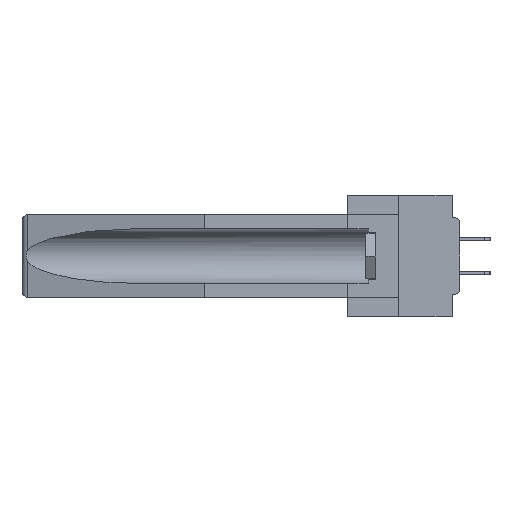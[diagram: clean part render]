
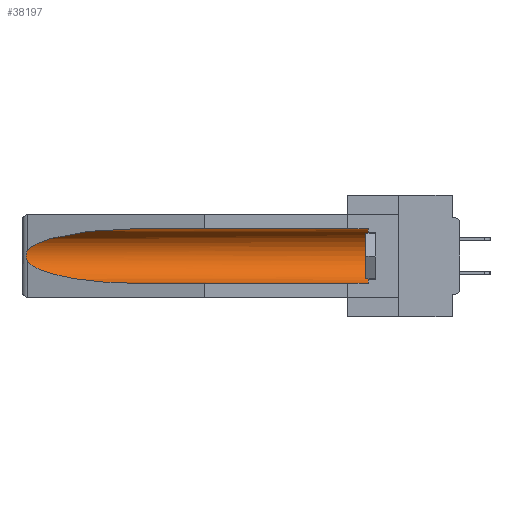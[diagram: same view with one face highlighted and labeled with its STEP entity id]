
A CAD part, left-side view. The second image highlights one B-rep face of the part: STEP entity #38197.
In plain terms, the highlighted cylindrical face has radius 2.857 mm (diameter 5.715 mm), a partial arc.
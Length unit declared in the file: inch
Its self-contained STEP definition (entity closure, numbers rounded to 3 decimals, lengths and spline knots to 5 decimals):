
#749 = CARTESIAN_POINT ( 'NONE',  ( 0.155, 0.126, -0.059 ) ) ;
#2860 = CARTESIAN_POINT ( 'NONE',  ( 0.25451, 1.48313, -0.09465 ) ) ;
#5526 = CARTESIAN_POINT ( 'NONE',  ( 0.2675, 1.53308, -0.16763 ) ) ;
#6172 = CARTESIAN_POINT ( 'NONE',  ( 0.26537, 1.52718, -0.14972 ) ) ;
#7469 = CARTESIAN_POINT ( 'NONE',  ( 0.155, 0.126, -0.1715 ) ) ;
#7649 = ORIENTED_EDGE ( 'NONE', *, *, #25995, .T. ) ;
#9247 = FACE_OUTER_BOUND ( 'NONE', #11034, .T. ) ;
#9677 = EDGE_CURVE ( 'NONE', #30293, #32261, #29166, .T. ) ;
#11034 = EDGE_LOOP ( 'NONE', ( #7649, #43003, #21508, #26777, #19174, #17220 ) ) ;
#11439 = VERTEX_POINT ( 'NONE', #749 ) ;
#12349 = VERTEX_POINT ( 'NONE', #33799 ) ;
#13702 = CARTESIAN_POINT ( 'NONE',  ( 0.155, 1.07973, -0.284 ) ) ;
#16605 = VERTEX_POINT ( 'NONE', #41737 ) ;
#17220 = ORIENTED_EDGE ( 'NONE', *, *, #38692, .T. ) ;
#17926 = DIRECTION ( 'NONE',  ( 0., -1., 0. ) ) ;
#17949 = AXIS2_PLACEMENT_3D ( 'NONE', #36084, #39409, #43514 ) ;
#19174 = ORIENTED_EDGE ( 'NONE', *, *, #40276, .T. ) ;
#19902 = CARTESIAN_POINT ( 'NONE',  ( 0.26597, 1.52961, -0.15275 ) ) ;
#20044 = CARTESIAN_POINT ( 'NONE',  ( 0.2673, 1.53269, -0.17917 ) ) ;
#20825 =( BOUNDED_CURVE ( )  B_SPLINE_CURVE ( 3, ( #22309, #40988, #26269, #29929 ),
 .UNSPECIFIED., .F., .F. ) 
 B_SPLINE_CURVE_WITH_KNOTS ( ( 4, 4 ),
 ( 0.1948, 1.5708 ),
 .UNSPECIFIED. ) 
 CURVE ( )  GEOMETRIC_REPRESENTATION_ITEM ( )  RATIONAL_B_SPLINE_CURVE ( ( 1., 0.848, 0.848, 1. ) ) 
 REPRESENTATION_ITEM ( '' )  );
#21004 = AXIS2_PLACEMENT_3D ( 'NONE', #7469, #17926, #43242 ) ;
#21508 = ORIENTED_EDGE ( 'NONE', *, *, #30151, .T. ) ;
#22309 = CARTESIAN_POINT ( 'NONE',  ( 0.26537, 1.52718, -0.19328 ) ) ;
#23246 = CARTESIAN_POINT ( 'NONE',  ( 0.21114, 1.30732, -0.059 ) ) ;
#23545 = CARTESIAN_POINT ( 'NONE',  ( 0.26654, 1.53092, -0.15636 ) ) ;
#23865 = CARTESIAN_POINT ( 'NONE',  ( 0.26597, 1.5296, -0.19026 ) ) ;
#24144 = CARTESIAN_POINT ( 'NONE',  ( 0.26537, 1.52718, -0.19328 ) ) ;
#25995 = EDGE_CURVE ( 'NONE', #12349, #16605, #44601, .T. ) ;
#26269 = CARTESIAN_POINT ( 'NONE',  ( 0.21114, 1.30732, -0.284 ) ) ;
#26777 = ORIENTED_EDGE ( 'NONE', *, *, #9677, .F. ) ;
#27198 = CARTESIAN_POINT ( 'NONE',  ( 0.2673, 1.5327, -0.16383 ) ) ;
#27356 = CARTESIAN_POINT ( 'NONE',  ( 0.26537, 1.52718, -0.19328 ) ) ;
#27520 = CARTESIAN_POINT ( 'NONE',  ( 0.26537, 1.52718, -0.14972 ) ) ;
#29166 = LINE ( 'NONE', #36547, #44927 ) ;
#29929 = CARTESIAN_POINT ( 'NONE',  ( 0.155, 1.07973, -0.284 ) ) ;
#30078 = CARTESIAN_POINT ( 'NONE',  ( 0.155, 0.126, -0.284 ) ) ;
#30151 = EDGE_CURVE ( 'NONE', #35829, #32261, #20825, .T. ) ;
#30293 = VERTEX_POINT ( 'NONE', #30078 ) ;
#31934 = CYLINDRICAL_SURFACE ( 'NONE', #17949, 0.1125 ) ;
#32261 = VERTEX_POINT ( 'NONE', #13702 ) ;
#33546 = LINE ( 'NONE', #46269, #35819 ) ;
#33799 = CARTESIAN_POINT ( 'NONE',  ( 0.155, 1.07973, -0.059 ) ) ;
#34497 = CARTESIAN_POINT ( 'NONE',  ( 0.2675, 1.53308, -0.17534 ) ) ;
#35560 = CIRCLE ( 'NONE', #21004, 0.1125 ) ;
#35819 = VECTOR ( 'NONE', #39165, 39.37008 ) ;
#35829 = VERTEX_POINT ( 'NONE', #24144 ) ;
#36084 = CARTESIAN_POINT ( 'NONE',  ( 0.155, -0.30754, -0.1715 ) ) ;
#36547 = CARTESIAN_POINT ( 'NONE',  ( 0.155, -0.30754, -0.284 ) ) ;
#38197 = ADVANCED_FACE ( 'NONE', ( #9247 ), #31934, .F. ) ;
#38692 = EDGE_CURVE ( 'NONE', #11439, #12349, #33546, .T. ) ;
#39165 = DIRECTION ( 'NONE',  ( 0., 1., 0. ) ) ;
#39409 = DIRECTION ( 'NONE',  ( 0., 1., 0. ) ) ;
#40276 = EDGE_CURVE ( 'NONE', #30293, #11439, #35560, .T. ) ;
#40988 = CARTESIAN_POINT ( 'NONE',  ( 0.25451, 1.48313, -0.24835 ) ) ;
#41168 = B_SPLINE_CURVE_WITH_KNOTS ( 'NONE', 3,
 ( #27520, #19902, #23545, #27198, #5526, #34497, #20044, #45374, #23865, #27356 ),
 .UNSPECIFIED., .F., .F.,
 ( 4, 2, 2, 2, 4 ),
 ( 0., 0.00029, 0.00058, 0.00087, 0.00117 ),
 .UNSPECIFIED. ) ;
#41481 = CARTESIAN_POINT ( 'NONE',  ( 0.155, 1.07973, -0.059 ) ) ;
#41737 = CARTESIAN_POINT ( 'NONE',  ( 0.26537, 1.52718, -0.14972 ) ) ;
#42175 = EDGE_CURVE ( 'NONE', #16605, #35829, #41168, .T. ) ;
#43003 = ORIENTED_EDGE ( 'NONE', *, *, #42175, .T. ) ;
#43242 = DIRECTION ( 'NONE',  ( 0., 0., 1. ) ) ;
#43347 = DIRECTION ( 'NONE',  ( 0., 1., 0. ) ) ;
#43514 = DIRECTION ( 'NONE',  ( 0., 0., 1. ) ) ;
#44601 =( BOUNDED_CURVE ( )  B_SPLINE_CURVE ( 3, ( #41481, #23246, #2860, #6172 ),
 .UNSPECIFIED., .F., .F. ) 
 B_SPLINE_CURVE_WITH_KNOTS ( ( 4, 4 ),
 ( 4.71239, 6.08839 ),
 .UNSPECIFIED. ) 
 CURVE ( )  GEOMETRIC_REPRESENTATION_ITEM ( )  RATIONAL_B_SPLINE_CURVE ( ( 1., 0.848, 0.848, 1. ) ) 
 REPRESENTATION_ITEM ( '' )  );
#44927 = VECTOR ( 'NONE', #43347, 39.37008 ) ;
#45374 = CARTESIAN_POINT ( 'NONE',  ( 0.26655, 1.53094, -0.18657 ) ) ;
#46269 = CARTESIAN_POINT ( 'NONE',  ( 0.155, -0.30754, -0.059 ) ) ;
